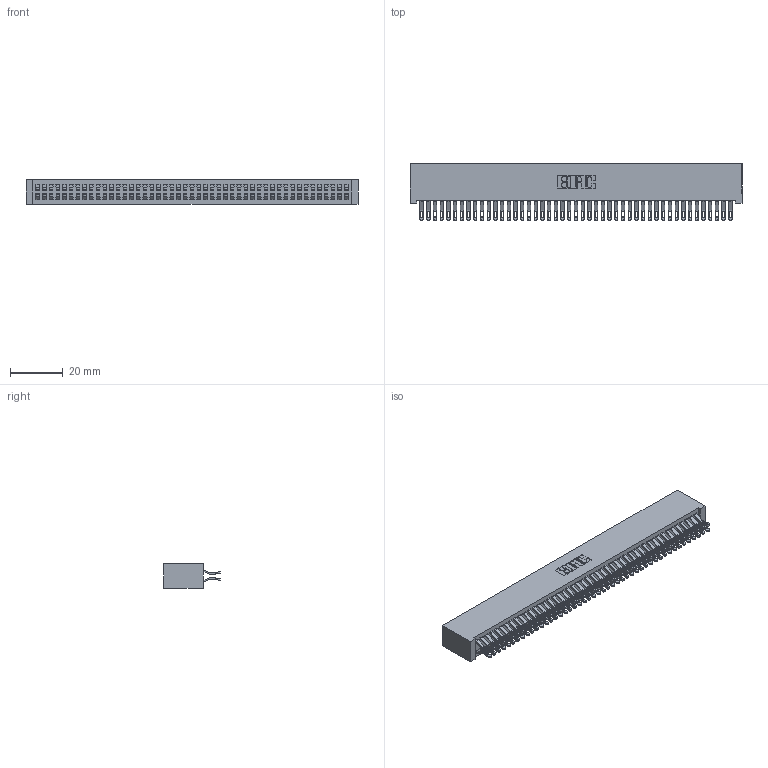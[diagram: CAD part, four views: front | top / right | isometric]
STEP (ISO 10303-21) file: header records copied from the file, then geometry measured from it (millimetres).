
FILE_DESCRIPTION (( 'STEP AP203' ), '1' );
FILE_NAME ('342-094-555-201.STEP', '2019-10-04T15:35:26', ( '' ), ( '' ), 'SwSTEP 2.0', 'SolidWorks 2016', '' );
FILE_SCHEMA (( 'CONFIG_CONTROL_DESIGN' ));
Length unit declared in the file: inch
Products named in the file (3): 342 Part_Lugless; 345-292-001_555 Tail; 342-094-555-201
Assembly tree (95 placements, depth 2):
  342-094-555-201
    342 Part_Lugless
    345-292-001_555 Tail  x94
Bounding box: 125.63 x 21.47 x 9.4 mm (x, y, z)
Volume: 12012.1 mm3; surface area: 21031.6 mm2
Topology: 95 solids, 95 shells, 5554 faces, 17477 edges, 11650 vertices
Faces by surface type: plane 3258, cylinder 2296
Entity records: 29507 total; most frequent: CARTESIAN_POINT 4916, ORIENTED_EDGE 4822, DIRECTION 4155, EDGE_CURVE 2411, VECTOR 2271, LINE 2271, VERTEX_POINT 1606, AXIS2_PLACEMENT_3D 942
